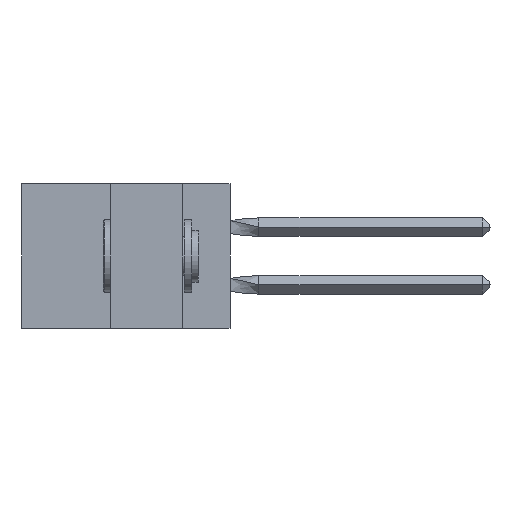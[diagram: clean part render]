
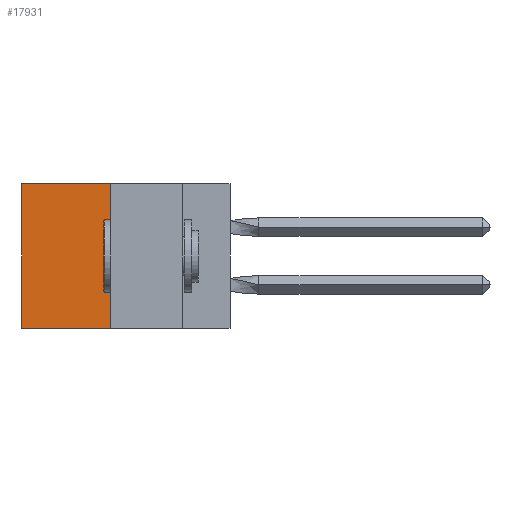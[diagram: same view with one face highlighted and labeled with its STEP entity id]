
A CAD part, left-side view. The second image highlights one B-rep face of the part: STEP entity #17931.
In plain terms, the highlighted planar face has unit normal (-1, 0, 0).
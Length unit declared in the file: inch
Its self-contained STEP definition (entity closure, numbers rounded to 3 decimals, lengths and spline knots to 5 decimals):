
#2810 = FACE_OUTER_BOUND ( 'NONE', #35300, .T. ) ;
#3264 = DIRECTION ( 'NONE',  ( 1., 0., 0. ) ) ;
#3393 = CARTESIAN_POINT ( 'NONE',  ( 0.305, 0.413, -0.5 ) ) ;
#5502 = VERTEX_POINT ( 'NONE', #27030 ) ;
#7904 = EDGE_CURVE ( 'NONE', #17203, #5502, #36872, .T. ) ;
#9567 = DIRECTION ( 'NONE',  ( 0., 0., -1. ) ) ;
#10182 = VECTOR ( 'NONE', #33269, 39.37008 ) ;
#11953 = VERTEX_POINT ( 'NONE', #12968 ) ;
#12707 = EDGE_CURVE ( 'NONE', #11953, #17203, #32396, .T. ) ;
#12968 = CARTESIAN_POINT ( 'NONE',  ( 0.305, 0.413, 0. ) ) ;
#15240 = DIRECTION ( 'NONE',  ( 0., 0., -1. ) ) ;
#15257 = DIRECTION ( 'NONE',  ( 0., 1., 0. ) ) ;
#17203 = VERTEX_POINT ( 'NONE', #25022 ) ;
#17439 = VECTOR ( 'NONE', #15240, 39.37008 ) ;
#17710 = ORIENTED_EDGE ( 'NONE', *, *, #22984, .T. ) ;
#17931 = ADVANCED_FACE ( 'NONE', ( #2810 ), #18699, .F. ) ;
#18699 = PLANE ( 'NONE',  #25087 ) ;
#19591 = ORIENTED_EDGE ( 'NONE', *, *, #29868, .T. ) ;
#20089 = LINE ( 'NONE', #30256, #24296 ) ;
#20163 = ORIENTED_EDGE ( 'NONE', *, *, #12707, .F. ) ;
#22926 = VERTEX_POINT ( 'NONE', #35598 ) ;
#22984 = EDGE_CURVE ( 'NONE', #11953, #22926, #20089, .T. ) ;
#23251 = DIRECTION ( 'NONE',  ( 0., 1., 0. ) ) ;
#24296 = VECTOR ( 'NONE', #15257, 39.37008 ) ;
#24555 = VECTOR ( 'NONE', #23251, 39.37008 ) ;
#25022 = CARTESIAN_POINT ( 'NONE',  ( 0.305, 0.413, -0.5 ) ) ;
#25087 = AXIS2_PLACEMENT_3D ( 'NONE', #3393, #3264, #9567 ) ;
#27030 = CARTESIAN_POINT ( 'NONE',  ( 0.305, 0.72, -0.5 ) ) ;
#29027 = ORIENTED_EDGE ( 'NONE', *, *, #7904, .F. ) ;
#29868 = EDGE_CURVE ( 'NONE', #22926, #5502, #38681, .T. ) ;
#30256 = CARTESIAN_POINT ( 'NONE',  ( 0.305, 0.413, 0. ) ) ;
#32396 = LINE ( 'NONE', #36210, #10182 ) ;
#32627 = CARTESIAN_POINT ( 'NONE',  ( 0.305, 0.413, -0.5 ) ) ;
#33165 = CARTESIAN_POINT ( 'NONE',  ( 0.305, 0.72, -0.5 ) ) ;
#33269 = DIRECTION ( 'NONE',  ( 0., 0., -1. ) ) ;
#35300 = EDGE_LOOP ( 'NONE', ( #19591, #29027, #20163, #17710 ) ) ;
#35598 = CARTESIAN_POINT ( 'NONE',  ( 0.305, 0.72, 0. ) ) ;
#36210 = CARTESIAN_POINT ( 'NONE',  ( 0.305, 0.413, -0.5 ) ) ;
#36872 = LINE ( 'NONE', #32627, #24555 ) ;
#38681 = LINE ( 'NONE', #33165, #17439 ) ;
